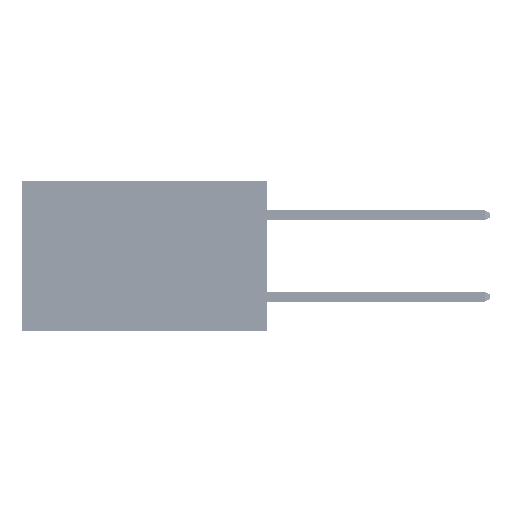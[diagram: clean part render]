
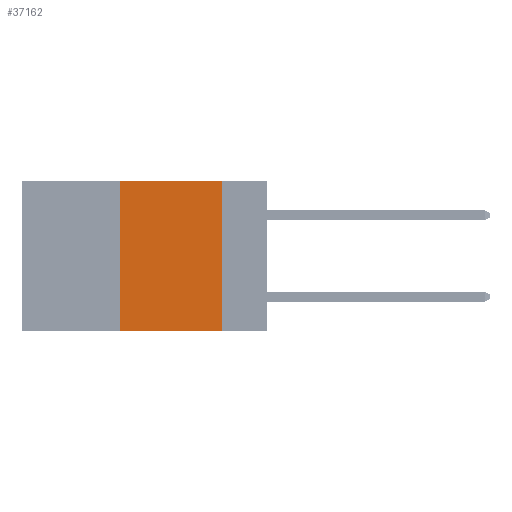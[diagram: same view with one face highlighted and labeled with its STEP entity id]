
A CAD part, left-side view. The second image highlights one B-rep face of the part: STEP entity #37162.
In plain terms, the highlighted planar face has unit normal (-1, 0, 0).
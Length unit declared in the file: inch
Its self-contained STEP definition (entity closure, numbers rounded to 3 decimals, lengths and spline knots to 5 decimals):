
#1646 = DIRECTION ( 'NONE',  ( 0., 0., -1. ) ) ;
#1830 = ORIENTED_EDGE ( 'NONE', *, *, #21674, .F. ) ;
#5001 = LINE ( 'NONE', #23071, #51423 ) ;
#5751 = VERTEX_POINT ( 'NONE', #32954 ) ;
#6663 = CARTESIAN_POINT ( 'NONE',  ( 0., 0.6, 0. ) ) ;
#7058 = DIRECTION ( 'NONE',  ( 0., 0., 1. ) ) ;
#8171 = VECTOR ( 'NONE', #1646, 39.37008 ) ;
#10416 = VERTEX_POINT ( 'NONE', #19030 ) ;
#13748 = VECTOR ( 'NONE', #14003, 39.37008 ) ;
#14003 = DIRECTION ( 'NONE',  ( 0., -1., 0. ) ) ;
#15198 = EDGE_CURVE ( 'NONE', #20306, #50131, #5001, .T. ) ;
#18134 = PLANE ( 'NONE',  #37892 ) ;
#19030 = CARTESIAN_POINT ( 'NONE',  ( 0., 0.11, 0. ) ) ;
#20306 = VERTEX_POINT ( 'NONE', #39936 ) ;
#21674 = EDGE_CURVE ( 'NONE', #50131, #10416, #38119, .T. ) ;
#22046 = LINE ( 'NONE', #34214, #13748 ) ;
#22065 = DIRECTION ( 'NONE',  ( 0., 0., -1. ) ) ;
#22151 = LINE ( 'NONE', #38266, #8171 ) ;
#22201 = EDGE_CURVE ( 'NONE', #10416, #5751, #22151, .T. ) ;
#22595 = EDGE_CURVE ( 'NONE', #20306, #5751, #22046, .T. ) ;
#23071 = CARTESIAN_POINT ( 'NONE',  ( 0., 0.36, 0. ) ) ;
#23452 = ORIENTED_EDGE ( 'NONE', *, *, #22201, .F. ) ;
#28703 = EDGE_LOOP ( 'NONE', ( #23452, #1830, #43268, #31438 ) ) ;
#29164 = VECTOR ( 'NONE', #42769, 39.37008 ) ;
#31438 = ORIENTED_EDGE ( 'NONE', *, *, #22595, .T. ) ;
#32954 = CARTESIAN_POINT ( 'NONE',  ( 0., 0.11, -0.37 ) ) ;
#34114 = CARTESIAN_POINT ( 'NONE',  ( 0., 0.6, 0. ) ) ;
#34214 = CARTESIAN_POINT ( 'NONE',  ( 0., 0.6, -0.37 ) ) ;
#37162 = ADVANCED_FACE ( 'NONE', ( #49755 ), #18134, .F. ) ;
#37892 = AXIS2_PLACEMENT_3D ( 'NONE', #34114, #50338, #22065 ) ;
#38119 = LINE ( 'NONE', #6663, #29164 ) ;
#38266 = CARTESIAN_POINT ( 'NONE',  ( 0., 0.11, 0. ) ) ;
#39936 = CARTESIAN_POINT ( 'NONE',  ( 0., 0.36, -0.37 ) ) ;
#42769 = DIRECTION ( 'NONE',  ( 0., -1., 0. ) ) ;
#43268 = ORIENTED_EDGE ( 'NONE', *, *, #15198, .F. ) ;
#49755 = FACE_OUTER_BOUND ( 'NONE', #28703, .T. ) ;
#50131 = VERTEX_POINT ( 'NONE', #50145 ) ;
#50145 = CARTESIAN_POINT ( 'NONE',  ( 0., 0.36, 0. ) ) ;
#50338 = DIRECTION ( 'NONE',  ( 1., 0., 0. ) ) ;
#51423 = VECTOR ( 'NONE', #7058, 39.37008 ) ;
